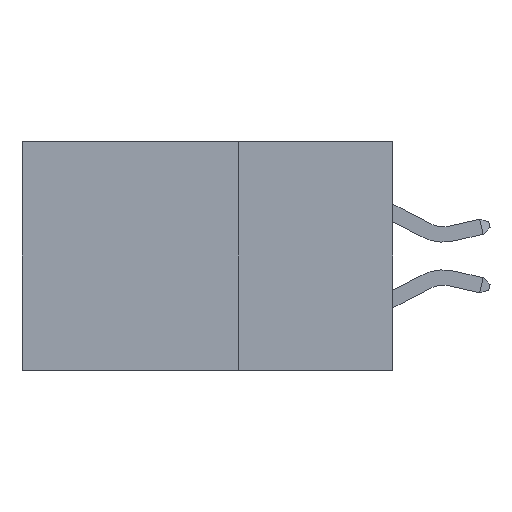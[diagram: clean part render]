
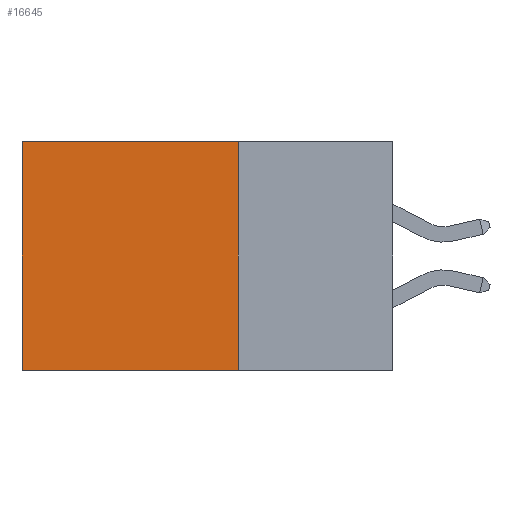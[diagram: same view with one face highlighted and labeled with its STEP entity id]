
A CAD part, left-side view. The second image highlights one B-rep face of the part: STEP entity #16645.
In plain terms, the highlighted planar face has unit normal (-1, 0, 0).
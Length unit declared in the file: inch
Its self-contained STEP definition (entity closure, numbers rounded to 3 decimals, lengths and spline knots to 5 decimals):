
#366 = EDGE_CURVE ( 'NONE', #8081, #17772, #5875, .T. ) ;
#746 = ORIENTED_EDGE ( 'NONE', *, *, #366, .F. ) ;
#1417 = VERTEX_POINT ( 'NONE', #37719 ) ;
#3197 = VECTOR ( 'NONE', #34571, 39.37008 ) ;
#4109 = CARTESIAN_POINT ( 'NONE',  ( 0.2875, 0.25, 0. ) ) ;
#5875 = LINE ( 'NONE', #12323, #21860 ) ;
#6696 = ORIENTED_EDGE ( 'NONE', *, *, #19306, .T. ) ;
#7309 = ORIENTED_EDGE ( 'NONE', *, *, #30745, .F. ) ;
#8081 = VERTEX_POINT ( 'NONE', #17840 ) ;
#10623 = DIRECTION ( 'NONE',  ( 1., 0., 0. ) ) ;
#11707 = CARTESIAN_POINT ( 'NONE',  ( 0.2875, 0.6, -0.37 ) ) ;
#12323 = CARTESIAN_POINT ( 'NONE',  ( 0.2875, 0.25, 0. ) ) ;
#13306 = LINE ( 'NONE', #17880, #15625 ) ;
#13538 = FACE_OUTER_BOUND ( 'NONE', #26298, .T. ) ;
#15625 = VECTOR ( 'NONE', #29064, 39.37008 ) ;
#16645 = ADVANCED_FACE ( 'NONE', ( #13538 ), #24952, .F. ) ;
#16764 = EDGE_CURVE ( 'NONE', #8081, #1417, #21980, .T. ) ;
#17772 = VERTEX_POINT ( 'NONE', #24687 ) ;
#17840 = CARTESIAN_POINT ( 'NONE',  ( 0.2875, 0.25, 0. ) ) ;
#17880 = CARTESIAN_POINT ( 'NONE',  ( 0.2875, 0.6, 0. ) ) ;
#18132 = DIRECTION ( 'NONE',  ( 0., 0., -1. ) ) ;
#19306 = EDGE_CURVE ( 'NONE', #1417, #35427, #13306, .T. ) ;
#20156 = ORIENTED_EDGE ( 'NONE', *, *, #16764, .T. ) ;
#21860 = VECTOR ( 'NONE', #18132, 39.37008 ) ;
#21980 = LINE ( 'NONE', #38705, #30450 ) ;
#24065 = AXIS2_PLACEMENT_3D ( 'NONE', #4109, #10623, #31640 ) ;
#24687 = CARTESIAN_POINT ( 'NONE',  ( 0.2875, 0.25, -0.37 ) ) ;
#24952 = PLANE ( 'NONE',  #24065 ) ;
#26228 = CARTESIAN_POINT ( 'NONE',  ( 0.2875, 0.25, -0.37 ) ) ;
#26298 = EDGE_LOOP ( 'NONE', ( #6696, #7309, #746, #20156 ) ) ;
#29064 = DIRECTION ( 'NONE',  ( 0., 0., -1. ) ) ;
#29792 = DIRECTION ( 'NONE',  ( 0., 1., 0. ) ) ;
#30070 = LINE ( 'NONE', #26228, #3197 ) ;
#30450 = VECTOR ( 'NONE', #29792, 39.37008 ) ;
#30745 = EDGE_CURVE ( 'NONE', #17772, #35427, #30070, .T. ) ;
#31640 = DIRECTION ( 'NONE',  ( 0., 0., -1. ) ) ;
#34571 = DIRECTION ( 'NONE',  ( 0., 1., 0. ) ) ;
#35427 = VERTEX_POINT ( 'NONE', #11707 ) ;
#37719 = CARTESIAN_POINT ( 'NONE',  ( 0.2875, 0.6, 0. ) ) ;
#38705 = CARTESIAN_POINT ( 'NONE',  ( 0.2875, 0.25, 0. ) ) ;
